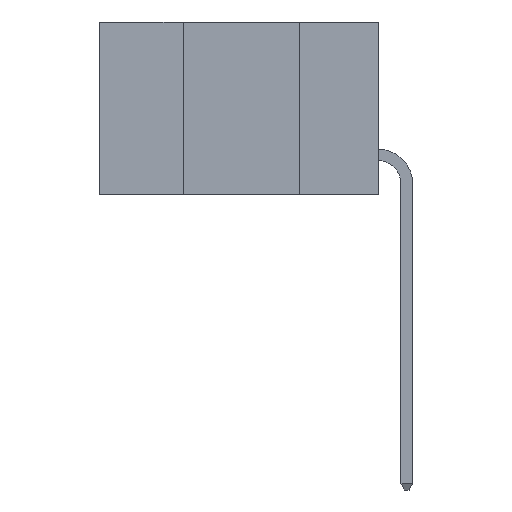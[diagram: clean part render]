
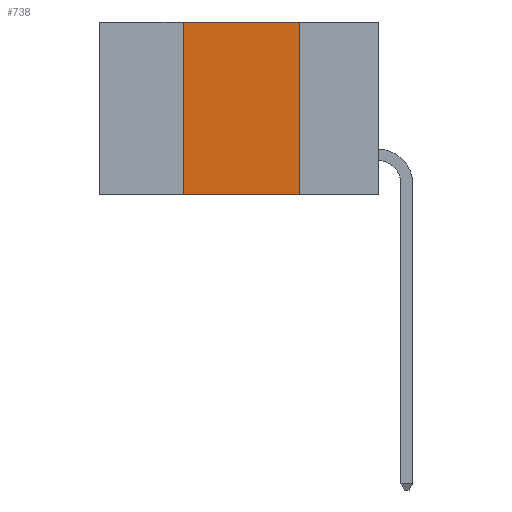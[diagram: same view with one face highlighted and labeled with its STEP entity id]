
A CAD part, left-side view. The second image highlights one B-rep face of the part: STEP entity #738.
In plain terms, the highlighted planar face has unit normal (-1, 0, 0).
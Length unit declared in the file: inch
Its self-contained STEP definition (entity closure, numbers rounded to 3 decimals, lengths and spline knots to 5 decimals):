
#637 = CARTESIAN_POINT ( 'NONE',  ( 0., 0.42, -0.37 ) ) ;
#738 = ADVANCED_FACE ( 'NONE', ( #5658 ), #12733, .F. ) ;
#1290 = EDGE_LOOP ( 'NONE', ( #9593, #10540, #10724, #9133 ) ) ;
#1642 = EDGE_CURVE ( 'NONE', #9192, #9489, #5403, .T. ) ;
#1804 = DIRECTION ( 'NONE',  ( 0., 0., 1. ) ) ;
#2142 = DIRECTION ( 'NONE',  ( 0., 0., -1. ) ) ;
#3248 = CARTESIAN_POINT ( 'NONE',  ( 0., 0.6, 0. ) ) ;
#3332 = CARTESIAN_POINT ( 'NONE',  ( 0., 0.17, -0.37 ) ) ;
#3753 = VERTEX_POINT ( 'NONE', #7789 ) ;
#4198 = DIRECTION ( 'NONE',  ( 0., -1., 0. ) ) ;
#4274 = CARTESIAN_POINT ( 'NONE',  ( 0., 0.17, -0.37 ) ) ;
#4615 = VERTEX_POINT ( 'NONE', #4274 ) ;
#4688 = VECTOR ( 'NONE', #12099, 39.37008 ) ;
#4737 = LINE ( 'NONE', #13783, #13109 ) ;
#5403 = LINE ( 'NONE', #10379, #7716 ) ;
#5658 = FACE_OUTER_BOUND ( 'NONE', #1290, .T. ) ;
#6083 = LINE ( 'NONE', #10349, #11470 ) ;
#6456 = AXIS2_PLACEMENT_3D ( 'NONE', #3248, #13837, #2142 ) ;
#6508 = EDGE_CURVE ( 'NONE', #3753, #4615, #9201, .T. ) ;
#7716 = VECTOR ( 'NONE', #1804, 39.37008 ) ;
#7789 = CARTESIAN_POINT ( 'NONE',  ( 0., 0.17, 0. ) ) ;
#8898 = EDGE_CURVE ( 'NONE', #9192, #4615, #4737, .T. ) ;
#9133 = ORIENTED_EDGE ( 'NONE', *, *, #8898, .T. ) ;
#9192 = VERTEX_POINT ( 'NONE', #637 ) ;
#9201 = LINE ( 'NONE', #3332, #4688 ) ;
#9489 = VERTEX_POINT ( 'NONE', #9845 ) ;
#9530 = DIRECTION ( 'NONE',  ( 0., -1., 0. ) ) ;
#9593 = ORIENTED_EDGE ( 'NONE', *, *, #6508, .F. ) ;
#9845 = CARTESIAN_POINT ( 'NONE',  ( 0., 0.42, 0. ) ) ;
#10349 = CARTESIAN_POINT ( 'NONE',  ( 0., 0.6, 0. ) ) ;
#10379 = CARTESIAN_POINT ( 'NONE',  ( 0., 0.42, -0.37 ) ) ;
#10540 = ORIENTED_EDGE ( 'NONE', *, *, #11312, .F. ) ;
#10724 = ORIENTED_EDGE ( 'NONE', *, *, #1642, .F. ) ;
#11312 = EDGE_CURVE ( 'NONE', #9489, #3753, #6083, .T. ) ;
#11470 = VECTOR ( 'NONE', #4198, 39.37008 ) ;
#12099 = DIRECTION ( 'NONE',  ( 0., 0., -1. ) ) ;
#12733 = PLANE ( 'NONE',  #6456 ) ;
#13109 = VECTOR ( 'NONE', #9530, 39.37008 ) ;
#13783 = CARTESIAN_POINT ( 'NONE',  ( 0., 0.6, -0.37 ) ) ;
#13837 = DIRECTION ( 'NONE',  ( 1., 0., 0. ) ) ;
